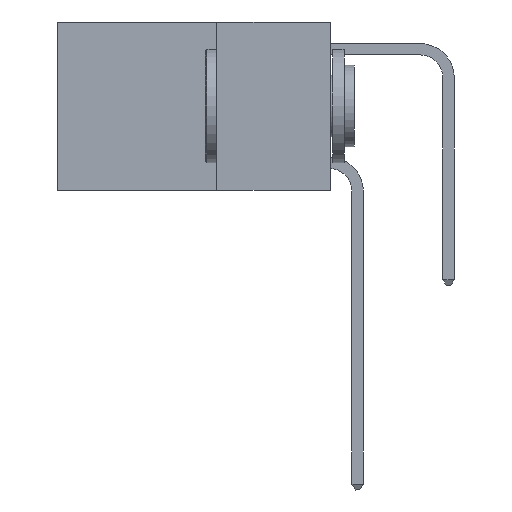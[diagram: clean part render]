
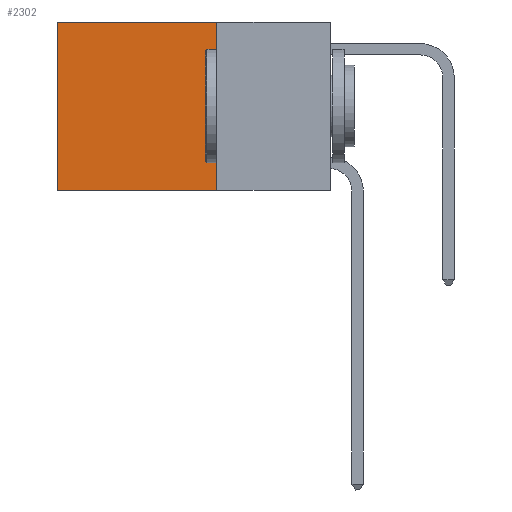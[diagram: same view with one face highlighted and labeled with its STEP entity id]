
A CAD part, left-side view. The second image highlights one B-rep face of the part: STEP entity #2302.
In plain terms, the highlighted planar face has unit normal (-1, 0, 0).
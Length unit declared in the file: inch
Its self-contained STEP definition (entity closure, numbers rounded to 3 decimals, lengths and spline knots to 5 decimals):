
#194 = FACE_OUTER_BOUND ( 'NONE', #3813, .T. ) ;
#338 = VERTEX_POINT ( 'NONE', #6529 ) ;
#476 = LINE ( 'NONE', #6874, #3678 ) ;
#594 = LINE ( 'NONE', #5387, #1650 ) ;
#1039 = CARTESIAN_POINT ( 'NONE',  ( 0.2625, 0.25, 0. ) ) ;
#1102 = DIRECTION ( 'NONE',  ( 0., 0., -1. ) ) ;
#1234 = EDGE_CURVE ( 'NONE', #338, #6420, #4115, .T. ) ;
#1428 = CARTESIAN_POINT ( 'NONE',  ( 0.2625, 0.25, -0.37 ) ) ;
#1650 = VECTOR ( 'NONE', #7983, 39.37008 ) ;
#2077 = ORIENTED_EDGE ( 'NONE', *, *, #2123, .F. ) ;
#2123 = EDGE_CURVE ( 'NONE', #9591, #8378, #4144, .T. ) ;
#2302 = ADVANCED_FACE ( 'NONE', ( #194 ), #8542, .F. ) ;
#3168 = CARTESIAN_POINT ( 'NONE',  ( 0.2625, 0.25, -0.37 ) ) ;
#3533 = CARTESIAN_POINT ( 'NONE',  ( 0.2625, 0.6, -0.37 ) ) ;
#3678 = VECTOR ( 'NONE', #7876, 39.37008 ) ;
#3813 = EDGE_LOOP ( 'NONE', ( #7176, #2077, #7415, #4408 ) ) ;
#4115 = LINE ( 'NONE', #7859, #6866 ) ;
#4144 = LINE ( 'NONE', #1428, #4653 ) ;
#4408 = ORIENTED_EDGE ( 'NONE', *, *, #1234, .T. ) ;
#4653 = VECTOR ( 'NONE', #7892, 39.37008 ) ;
#5387 = CARTESIAN_POINT ( 'NONE',  ( 0.2625, 0.25, 0. ) ) ;
#5410 = EDGE_CURVE ( 'NONE', #338, #9591, #594, .T. ) ;
#5791 = DIRECTION ( 'NONE',  ( 1., 0., 0. ) ) ;
#6420 = VERTEX_POINT ( 'NONE', #10393 ) ;
#6529 = CARTESIAN_POINT ( 'NONE',  ( 0.2625, 0.25, 0. ) ) ;
#6866 = VECTOR ( 'NONE', #11472, 39.37008 ) ;
#6874 = CARTESIAN_POINT ( 'NONE',  ( 0.2625, 0.6, 0. ) ) ;
#7176 = ORIENTED_EDGE ( 'NONE', *, *, #7993, .T. ) ;
#7415 = ORIENTED_EDGE ( 'NONE', *, *, #5410, .F. ) ;
#7859 = CARTESIAN_POINT ( 'NONE',  ( 0.2625, 0.25, 0. ) ) ;
#7876 = DIRECTION ( 'NONE',  ( 0., 0., -1. ) ) ;
#7892 = DIRECTION ( 'NONE',  ( 0., 1., 0. ) ) ;
#7983 = DIRECTION ( 'NONE',  ( 0., 0., -1. ) ) ;
#7993 = EDGE_CURVE ( 'NONE', #6420, #8378, #476, .T. ) ;
#8378 = VERTEX_POINT ( 'NONE', #3533 ) ;
#8542 = PLANE ( 'NONE',  #9012 ) ;
#9012 = AXIS2_PLACEMENT_3D ( 'NONE', #1039, #5791, #1102 ) ;
#9591 = VERTEX_POINT ( 'NONE', #3168 ) ;
#10393 = CARTESIAN_POINT ( 'NONE',  ( 0.2625, 0.6, 0. ) ) ;
#11472 = DIRECTION ( 'NONE',  ( 0., 1., 0. ) ) ;
